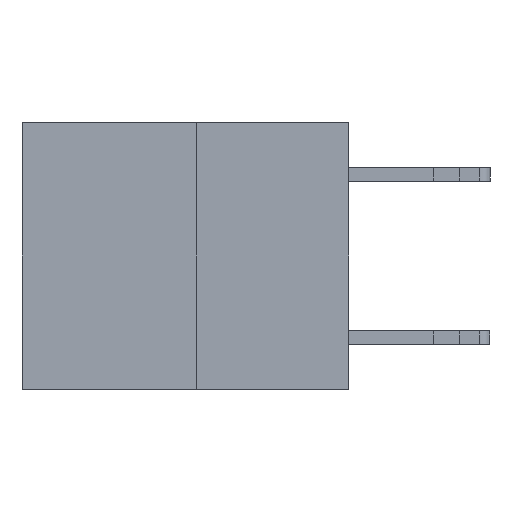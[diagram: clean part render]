
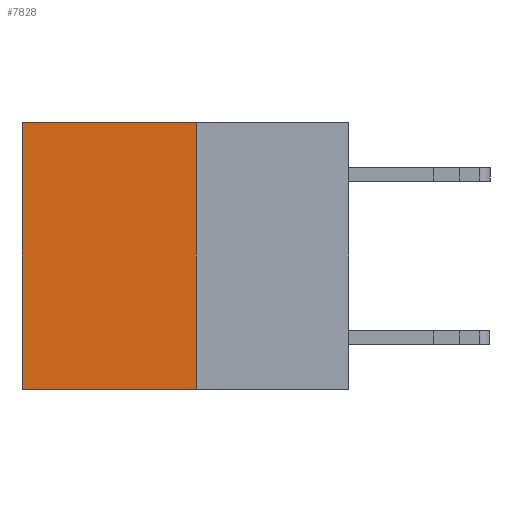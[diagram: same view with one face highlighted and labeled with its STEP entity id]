
A CAD part, left-side view. The second image highlights one B-rep face of the part: STEP entity #7828.
In plain terms, the highlighted planar face has unit normal (-1, 0, 0).
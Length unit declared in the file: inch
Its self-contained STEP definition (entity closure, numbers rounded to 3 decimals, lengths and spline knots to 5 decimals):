
#56 = DIRECTION ( 'NONE',  ( 0., 1., 0. ) ) ;
#529 = EDGE_CURVE ( 'NONE', #20157, #7465, #16891, .T. ) ;
#733 = CARTESIAN_POINT ( 'NONE',  ( 0.3165, 0.6, -0.49 ) ) ;
#1343 = VERTEX_POINT ( 'NONE', #14800 ) ;
#1678 = CARTESIAN_POINT ( 'NONE',  ( 0.3165, 0.28, -0.49 ) ) ;
#3392 = EDGE_CURVE ( 'NONE', #1343, #10246, #8361, .T. ) ;
#5100 = CARTESIAN_POINT ( 'NONE',  ( 0.3165, 0.28, 0. ) ) ;
#5244 = DIRECTION ( 'NONE',  ( 0., 1., 0. ) ) ;
#5413 = VECTOR ( 'NONE', #56, 39.37008 ) ;
#6532 = ORIENTED_EDGE ( 'NONE', *, *, #3392, .T. ) ;
#7465 = VERTEX_POINT ( 'NONE', #16120 ) ;
#7828 = ADVANCED_FACE ( 'NONE', ( #16334 ), #13559, .F. ) ;
#8361 = LINE ( 'NONE', #733, #13778 ) ;
#8716 = CARTESIAN_POINT ( 'NONE',  ( 0.3165, 0.28, -0.49 ) ) ;
#8848 = DIRECTION ( 'NONE',  ( 0., 0., -1. ) ) ;
#8913 = DIRECTION ( 'NONE',  ( 1., 0., 0. ) ) ;
#10196 = VECTOR ( 'NONE', #5244, 39.37008 ) ;
#10246 = VERTEX_POINT ( 'NONE', #14300 ) ;
#10359 = LINE ( 'NONE', #14062, #5413 ) ;
#10802 = EDGE_CURVE ( 'NONE', #7465, #10246, #10359, .T. ) ;
#11082 = AXIS2_PLACEMENT_3D ( 'NONE', #8716, #8913, #8848 ) ;
#11159 = DIRECTION ( 'NONE',  ( 0., 0., -1. ) ) ;
#12812 = EDGE_LOOP ( 'NONE', ( #6532, #13572, #17273, #18027 ) ) ;
#13382 = DIRECTION ( 'NONE',  ( 0., 0., -1. ) ) ;
#13559 = PLANE ( 'NONE',  #11082 ) ;
#13572 = ORIENTED_EDGE ( 'NONE', *, *, #10802, .F. ) ;
#13778 = VECTOR ( 'NONE', #13382, 39.37008 ) ;
#14062 = CARTESIAN_POINT ( 'NONE',  ( 0.3165, 0.28, -0.49 ) ) ;
#14300 = CARTESIAN_POINT ( 'NONE',  ( 0.3165, 0.6, -0.49 ) ) ;
#14375 = LINE ( 'NONE', #5100, #10196 ) ;
#14631 = CARTESIAN_POINT ( 'NONE',  ( 0.3165, 0.28, 0. ) ) ;
#14758 = EDGE_CURVE ( 'NONE', #20157, #1343, #14375, .T. ) ;
#14800 = CARTESIAN_POINT ( 'NONE',  ( 0.3165, 0.6, 0. ) ) ;
#16120 = CARTESIAN_POINT ( 'NONE',  ( 0.3165, 0.28, -0.49 ) ) ;
#16334 = FACE_OUTER_BOUND ( 'NONE', #12812, .T. ) ;
#16891 = LINE ( 'NONE', #1678, #19575 ) ;
#17273 = ORIENTED_EDGE ( 'NONE', *, *, #529, .F. ) ;
#18027 = ORIENTED_EDGE ( 'NONE', *, *, #14758, .T. ) ;
#19575 = VECTOR ( 'NONE', #11159, 39.37008 ) ;
#20157 = VERTEX_POINT ( 'NONE', #14631 ) ;
